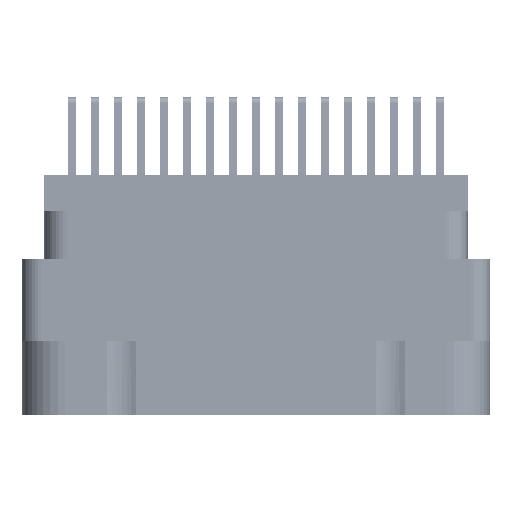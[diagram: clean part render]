
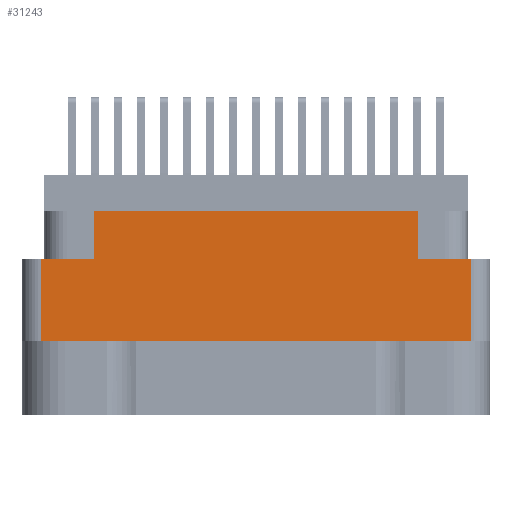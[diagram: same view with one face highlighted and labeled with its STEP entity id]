
A CAD part, left-side view. The second image highlights one B-rep face of the part: STEP entity #31243.
In plain terms, the highlighted planar face has unit normal (-1, 0, 0).
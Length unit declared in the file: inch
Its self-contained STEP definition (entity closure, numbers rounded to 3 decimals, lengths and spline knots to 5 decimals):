
#624 = ORIENTED_EDGE ( 'NONE', *, *, #15771, .F. ) ;
#660 = LINE ( 'NONE', #15186, #31259 ) ;
#1793 = VECTOR ( 'NONE', #75280, 39.37008 ) ;
#3580 = DIRECTION ( 'NONE',  ( 0., 0., 1. ) ) ;
#3748 = CARTESIAN_POINT ( 'NONE',  ( -1.375, -0.5285, -0.274 ) ) ;
#5212 = CARTESIAN_POINT ( 'NONE',  ( -1.375, -0.7005, -0.274 ) ) ;
#5224 = CARTESIAN_POINT ( 'NONE',  ( -1.375, -0.5285, -0.274 ) ) ;
#5519 = EDGE_LOOP ( 'NONE', ( #27773, #67987, #87672, #53296, #38318, #72457, #624, #25221 ) ) ;
#5581 = LINE ( 'NONE', #14518, #9941 ) ;
#6588 = DIRECTION ( 'NONE',  ( 0., 0., 1. ) ) ;
#6848 = VERTEX_POINT ( 'NONE', #77153 ) ;
#9781 = EDGE_CURVE ( 'NONE', #75323, #79915, #660, .T. ) ;
#9941 = VECTOR ( 'NONE', #77466, 39.37008 ) ;
#10885 = CARTESIAN_POINT ( 'NONE',  ( -1.375, -0.7005, -0.54 ) ) ;
#13311 = LINE ( 'NONE', #52593, #20903 ) ;
#13404 = CARTESIAN_POINT ( 'NONE',  ( -1.375, -0.7005, -0.78 ) ) ;
#14518 = CARTESIAN_POINT ( 'NONE',  ( -1.375, 0.7625, -0.117 ) ) ;
#15186 = CARTESIAN_POINT ( 'NONE',  ( -1.375, 0., -0.274 ) ) ;
#15771 = EDGE_CURVE ( 'NONE', #62667, #6848, #5581, .T. ) ;
#16896 = DIRECTION ( 'NONE',  ( 0., -1., 0. ) ) ;
#20903 = VECTOR ( 'NONE', #47056, 39.37008 ) ;
#22151 = DIRECTION ( 'NONE',  ( 0., 0., -1. ) ) ;
#23767 = DIRECTION ( 'NONE',  ( -1., 0., 0. ) ) ;
#25221 = ORIENTED_EDGE ( 'NONE', *, *, #72141, .F. ) ;
#26331 = VECTOR ( 'NONE', #56537, 39.37008 ) ;
#27398 = EDGE_CURVE ( 'NONE', #89943, #6848, #81648, .T. ) ;
#27736 = CARTESIAN_POINT ( 'NONE',  ( -1.375, 0.7005, -0.54 ) ) ;
#27773 = ORIENTED_EDGE ( 'NONE', *, *, #9781, .F. ) ;
#30389 = VERTEX_POINT ( 'NONE', #5212 ) ;
#31243 = ADVANCED_FACE ( 'NONE', ( #31342 ), #80031, .T. ) ;
#31259 = VECTOR ( 'NONE', #36519, 39.37008 ) ;
#31342 = FACE_OUTER_BOUND ( 'NONE', #5519, .T. ) ;
#36519 = DIRECTION ( 'NONE',  ( 0., -1., 0. ) ) ;
#38108 = CARTESIAN_POINT ( 'NONE',  ( -1.375, -0.7625, -0.78 ) ) ;
#38318 = ORIENTED_EDGE ( 'NONE', *, *, #72403, .F. ) ;
#39684 = VECTOR ( 'NONE', #22151, 39.37008 ) ;
#41377 = LINE ( 'NONE', #13404, #66507 ) ;
#43170 = AXIS2_PLACEMENT_3D ( 'NONE', #38108, #23767, #3580 ) ;
#46625 = VECTOR ( 'NONE', #16896, 39.37008 ) ;
#46672 = VERTEX_POINT ( 'NONE', #10885 ) ;
#47056 = DIRECTION ( 'NONE',  ( 0., -1., 0. ) ) ;
#51690 = CARTESIAN_POINT ( 'NONE',  ( -1.375, 0., -0.54 ) ) ;
#52593 = CARTESIAN_POINT ( 'NONE',  ( -1.375, 0., -0.274 ) ) ;
#53296 = ORIENTED_EDGE ( 'NONE', *, *, #53865, .T. ) ;
#53865 = EDGE_CURVE ( 'NONE', #46672, #30389, #41377, .T. ) ;
#53872 = VERTEX_POINT ( 'NONE', #27736 ) ;
#56537 = DIRECTION ( 'NONE',  ( 0., 0., 1. ) ) ;
#62667 = VERTEX_POINT ( 'NONE', #84809 ) ;
#66507 = VECTOR ( 'NONE', #6588, 39.37008 ) ;
#67987 = ORIENTED_EDGE ( 'NONE', *, *, #71142, .T. ) ;
#69934 = CARTESIAN_POINT ( 'NONE',  ( -1.375, 0.7005, -0.274 ) ) ;
#70077 = LINE ( 'NONE', #77136, #26331 ) ;
#70701 = CARTESIAN_POINT ( 'NONE',  ( -1.375, 0.7005, -0.78 ) ) ;
#71142 = EDGE_CURVE ( 'NONE', #75323, #53872, #80213, .T. ) ;
#72141 = EDGE_CURVE ( 'NONE', #79915, #62667, #70077, .T. ) ;
#72403 = EDGE_CURVE ( 'NONE', #89943, #30389, #13311, .T. ) ;
#72457 = ORIENTED_EDGE ( 'NONE', *, *, #27398, .T. ) ;
#75280 = DIRECTION ( 'NONE',  ( 0., 0., 1. ) ) ;
#75323 = VERTEX_POINT ( 'NONE', #69934 ) ;
#77136 = CARTESIAN_POINT ( 'NONE',  ( -1.375, 0.5285, -0.274 ) ) ;
#77153 = CARTESIAN_POINT ( 'NONE',  ( -1.375, -0.5285, -0.117 ) ) ;
#77466 = DIRECTION ( 'NONE',  ( 0., -1., 0. ) ) ;
#78699 = EDGE_CURVE ( 'NONE', #53872, #46672, #82683, .T. ) ;
#79202 = CARTESIAN_POINT ( 'NONE',  ( -1.375, 0.5285, -0.274 ) ) ;
#79915 = VERTEX_POINT ( 'NONE', #79202 ) ;
#80031 = PLANE ( 'NONE',  #43170 ) ;
#80213 = LINE ( 'NONE', #70701, #39684 ) ;
#81648 = LINE ( 'NONE', #5224, #1793 ) ;
#82683 = LINE ( 'NONE', #51690, #46625 ) ;
#84809 = CARTESIAN_POINT ( 'NONE',  ( -1.375, 0.5285, -0.117 ) ) ;
#87672 = ORIENTED_EDGE ( 'NONE', *, *, #78699, .T. ) ;
#89943 = VERTEX_POINT ( 'NONE', #3748 ) ;
